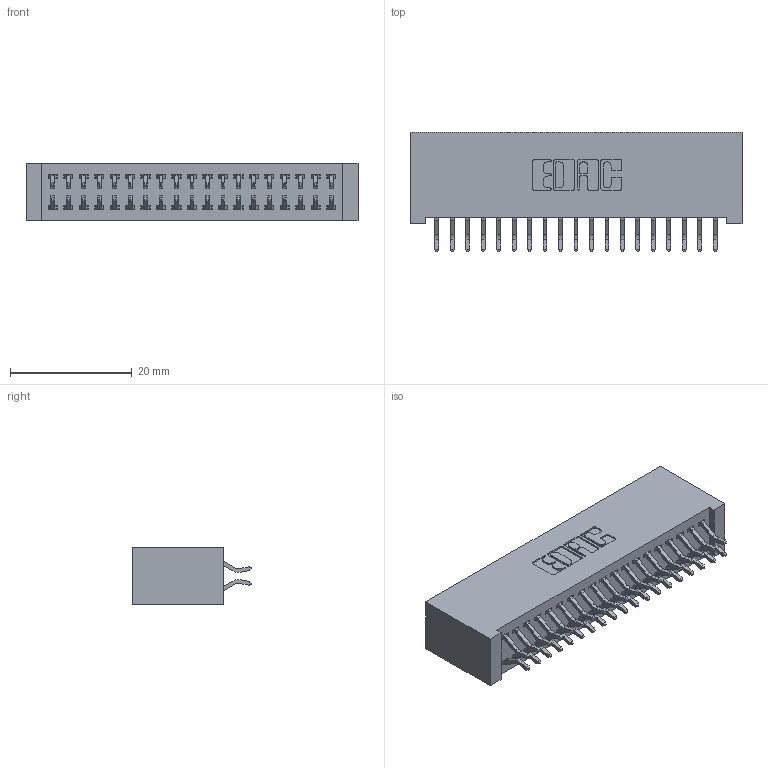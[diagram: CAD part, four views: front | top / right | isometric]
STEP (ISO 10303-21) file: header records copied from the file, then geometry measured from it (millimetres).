
FILE_DESCRIPTION (( 'STEP AP203' ), '1' );
FILE_NAME ('392-038-556-201.STEP', '2019-10-07T19:07:26', ( '' ), ( '' ), 'SwSTEP 2.0', 'SolidWorks 2016', '' );
FILE_SCHEMA (( 'CONFIG_CONTROL_DESIGN' ));
Length unit declared in the file: inch
Products named in the file (3): 392-038-556-201; 342 Part_Lugless; 345-292-001_556 Tail
Assembly tree (39 placements, depth 2):
  392-038-556-201
    342 Part_Lugless
    345-292-001_556 Tail  x38
Bounding box: 54.51 x 19.58 x 9.4 mm (x, y, z)
Volume: 5227.3 mm3; surface area: 8351.3 mm2
Topology: 39 solids, 39 shells, 2306 faces, 6849 edges, 4514 vertices
Faces by surface type: plane 1582, cylinder 724
Entity records: 15009 total; most frequent: CARTESIAN_POINT 2526, ORIENTED_EDGE 2450, DIRECTION 2181, EDGE_CURVE 1225, VECTOR 1097, LINE 1097, VERTEX_POINT 814, AXIS2_PLACEMENT_3D 542
